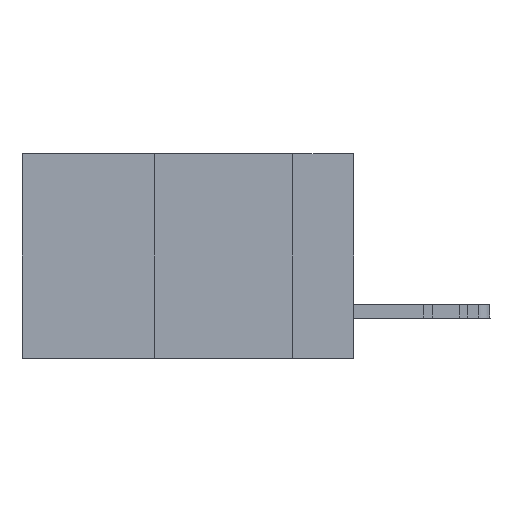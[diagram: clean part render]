
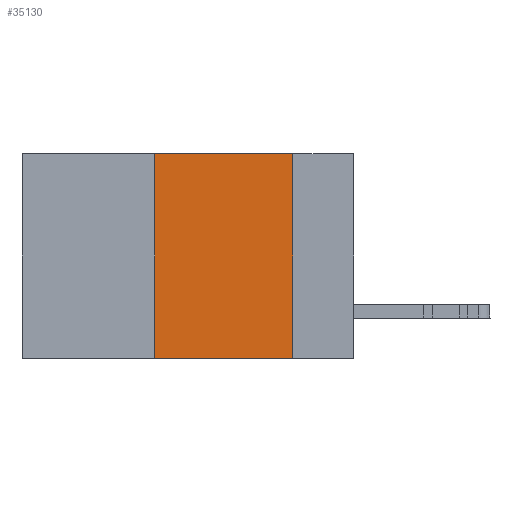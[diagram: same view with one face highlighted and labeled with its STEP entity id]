
A CAD part, left-side view. The second image highlights one B-rep face of the part: STEP entity #35130.
In plain terms, the highlighted planar face has unit normal (-1, 0, 0).
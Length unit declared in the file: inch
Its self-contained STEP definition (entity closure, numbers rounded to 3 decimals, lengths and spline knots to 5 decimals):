
#1308 = VERTEX_POINT ( 'NONE', #5701 ) ;
#2585 = DIRECTION ( 'NONE',  ( 0., -1., 0. ) ) ;
#3918 = LINE ( 'NONE', #24149, #18945 ) ;
#4664 = DIRECTION ( 'NONE',  ( 1., 0., 0. ) ) ;
#5701 = CARTESIAN_POINT ( 'NONE',  ( 0., 0.36, -0.37 ) ) ;
#6071 = LINE ( 'NONE', #15950, #13087 ) ;
#7777 = FACE_OUTER_BOUND ( 'NONE', #18796, .T. ) ;
#8987 = CARTESIAN_POINT ( 'NONE',  ( 0., 0.11, 0. ) ) ;
#10907 = DIRECTION ( 'NONE',  ( 0., 0., -1. ) ) ;
#13087 = VECTOR ( 'NONE', #32629, 39.37008 ) ;
#13807 = ORIENTED_EDGE ( 'NONE', *, *, #24295, .F. ) ;
#13826 = EDGE_CURVE ( 'NONE', #1308, #38944, #3918, .T. ) ;
#15738 = CARTESIAN_POINT ( 'NONE',  ( 0., 0.36, 0. ) ) ;
#15742 = EDGE_CURVE ( 'NONE', #1308, #23448, #6071, .T. ) ;
#15950 = CARTESIAN_POINT ( 'NONE',  ( 0., 0.36, 0. ) ) ;
#17070 = EDGE_CURVE ( 'NONE', #22965, #38944, #20982, .T. ) ;
#18796 = EDGE_LOOP ( 'NONE', ( #33849, #13807, #36528, #37761 ) ) ;
#18945 = VECTOR ( 'NONE', #37538, 39.37008 ) ;
#20982 = LINE ( 'NONE', #27578, #33688 ) ;
#22965 = VERTEX_POINT ( 'NONE', #8987 ) ;
#23448 = VERTEX_POINT ( 'NONE', #15738 ) ;
#24149 = CARTESIAN_POINT ( 'NONE',  ( 0., 0.6, -0.37 ) ) ;
#24295 = EDGE_CURVE ( 'NONE', #23448, #22965, #39907, .T. ) ;
#24680 = DIRECTION ( 'NONE',  ( 0., 0., -1. ) ) ;
#24972 = VECTOR ( 'NONE', #2585, 39.37008 ) ;
#27578 = CARTESIAN_POINT ( 'NONE',  ( 0., 0.11, 0. ) ) ;
#28615 = CARTESIAN_POINT ( 'NONE',  ( 0., 0.6, 0. ) ) ;
#29964 = AXIS2_PLACEMENT_3D ( 'NONE', #28615, #4664, #24680 ) ;
#32629 = DIRECTION ( 'NONE',  ( 0., 0., 1. ) ) ;
#33688 = VECTOR ( 'NONE', #10907, 39.37008 ) ;
#33849 = ORIENTED_EDGE ( 'NONE', *, *, #17070, .F. ) ;
#34723 = CARTESIAN_POINT ( 'NONE',  ( 0., 0.11, -0.37 ) ) ;
#35130 = ADVANCED_FACE ( 'NONE', ( #7777 ), #41986, .F. ) ;
#36528 = ORIENTED_EDGE ( 'NONE', *, *, #15742, .F. ) ;
#37538 = DIRECTION ( 'NONE',  ( 0., -1., 0. ) ) ;
#37761 = ORIENTED_EDGE ( 'NONE', *, *, #13826, .T. ) ;
#38944 = VERTEX_POINT ( 'NONE', #34723 ) ;
#39907 = LINE ( 'NONE', #43136, #24972 ) ;
#41986 = PLANE ( 'NONE',  #29964 ) ;
#43136 = CARTESIAN_POINT ( 'NONE',  ( 0., 0.6, 0. ) ) ;
